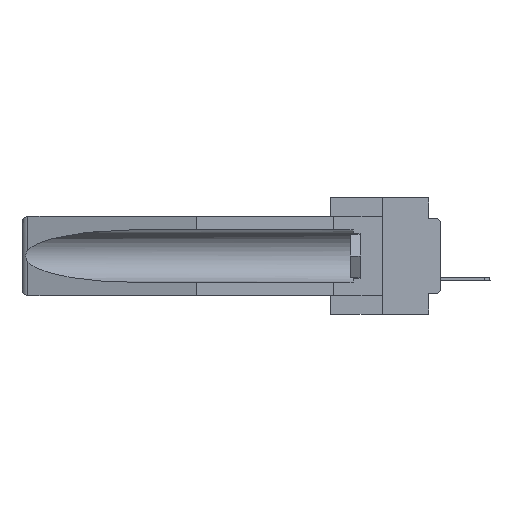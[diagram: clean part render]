
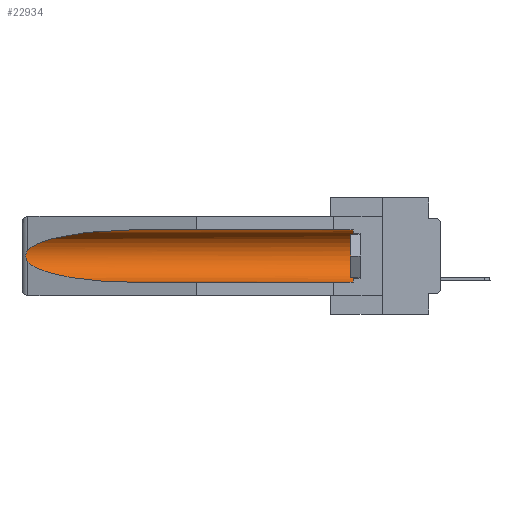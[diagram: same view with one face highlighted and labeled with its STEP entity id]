
A CAD part, left-side view. The second image highlights one B-rep face of the part: STEP entity #22934.
In plain terms, the highlighted cylindrical face has radius 2.857 mm (diameter 5.715 mm), a partial arc.
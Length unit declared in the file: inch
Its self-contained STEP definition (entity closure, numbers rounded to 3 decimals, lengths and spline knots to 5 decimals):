
#300 = CARTESIAN_POINT ( 'NONE',  ( 0.2675, 1.53308, -0.16763 ) ) ;
#750 = DIRECTION ( 'NONE',  ( 0., 0., 1. ) ) ;
#2092 = DIRECTION ( 'NONE',  ( 0., 1., 0. ) ) ;
#3161 = CARTESIAN_POINT ( 'NONE',  ( 0.2673, 1.53269, -0.17917 ) ) ;
#3666 = CARTESIAN_POINT ( 'NONE',  ( 0.26654, 1.53092, -0.15636 ) ) ;
#3973 = CARTESIAN_POINT ( 'NONE',  ( 0.21114, 1.30732, -0.284 ) ) ;
#4116 = VECTOR ( 'NONE', #8752, 39.37008 ) ;
#5172 = ORIENTED_EDGE ( 'NONE', *, *, #27428, .F. ) ;
#6545 = CARTESIAN_POINT ( 'NONE',  ( 0.26597, 1.5296, -0.19026 ) ) ;
#8145 = AXIS2_PLACEMENT_3D ( 'NONE', #26510, #17814, #750 ) ;
#8363 = ORIENTED_EDGE ( 'NONE', *, *, #35321, .T. ) ;
#8752 = DIRECTION ( 'NONE',  ( 0., 1., 0. ) ) ;
#10438 = CARTESIAN_POINT ( 'NONE',  ( 0.26537, 1.52718, -0.14972 ) ) ;
#11180 = CARTESIAN_POINT ( 'NONE',  ( 0.155, 0.126, -0.284 ) ) ;
#11376 = EDGE_CURVE ( 'NONE', #19809, #11511, #11551, .T. ) ;
#11491 = VERTEX_POINT ( 'NONE', #33739 ) ;
#11511 = VERTEX_POINT ( 'NONE', #22218 ) ;
#11551 =( BOUNDED_CURVE ( )  B_SPLINE_CURVE ( 3, ( #33262, #36137, #21859, #10438 ),
 .UNSPECIFIED., .F., .F. ) 
 B_SPLINE_CURVE_WITH_KNOTS ( ( 4, 4 ),
 ( 4.71239, 6.08839 ),
 .UNSPECIFIED. ) 
 CURVE ( )  GEOMETRIC_REPRESENTATION_ITEM ( )  RATIONAL_B_SPLINE_CURVE ( ( 1., 0.848, 0.848, 1. ) ) 
 REPRESENTATION_ITEM ( '' )  );
#12592 = CARTESIAN_POINT ( 'NONE',  ( 0.25451, 1.48313, -0.24835 ) ) ;
#12734 =( BOUNDED_CURVE ( )  B_SPLINE_CURVE ( 3, ( #32417, #12592, #3973, #29912 ),
 .UNSPECIFIED., .F., .F. ) 
 B_SPLINE_CURVE_WITH_KNOTS ( ( 4, 4 ),
 ( 0.1948, 1.5708 ),
 .UNSPECIFIED. ) 
 CURVE ( )  GEOMETRIC_REPRESENTATION_ITEM ( )  RATIONAL_B_SPLINE_CURVE ( ( 1., 0.848, 0.848, 1. ) ) 
 REPRESENTATION_ITEM ( '' )  );
#12926 = VERTEX_POINT ( 'NONE', #34328 ) ;
#13535 = CARTESIAN_POINT ( 'NONE',  ( 0.155, -0.30754, -0.059 ) ) ;
#14119 = VERTEX_POINT ( 'NONE', #20890 ) ;
#14745 = CARTESIAN_POINT ( 'NONE',  ( 0.26597, 1.52961, -0.15275 ) ) ;
#14881 = CARTESIAN_POINT ( 'NONE',  ( 0.26655, 1.53094, -0.18657 ) ) ;
#16015 = ORIENTED_EDGE ( 'NONE', *, *, #17684, .T. ) ;
#16871 = LINE ( 'NONE', #13535, #22609 ) ;
#17504 = EDGE_LOOP ( 'NONE', ( #25934, #35604, #16015, #5172, #17591, #8363 ) ) ;
#17591 = ORIENTED_EDGE ( 'NONE', *, *, #36355, .T. ) ;
#17625 = CARTESIAN_POINT ( 'NONE',  ( 0.26537, 1.52718, -0.19328 ) ) ;
#17684 = EDGE_CURVE ( 'NONE', #12926, #11491, #12734, .T. ) ;
#17814 = DIRECTION ( 'NONE',  ( 0., -1., 0. ) ) ;
#19809 = VERTEX_POINT ( 'NONE', #33232 ) ;
#20115 = LINE ( 'NONE', #27260, #4116 ) ;
#20890 = CARTESIAN_POINT ( 'NONE',  ( 0.155, 0.126, -0.059 ) ) ;
#21670 = CIRCLE ( 'NONE', #8145, 0.1125 ) ;
#21859 = CARTESIAN_POINT ( 'NONE',  ( 0.25451, 1.48313, -0.09465 ) ) ;
#22218 = CARTESIAN_POINT ( 'NONE',  ( 0.26537, 1.52718, -0.14972 ) ) ;
#22609 = VECTOR ( 'NONE', #2092, 39.37008 ) ;
#22934 = ADVANCED_FACE ( 'NONE', ( #25501 ), #28651, .F. ) ;
#23384 = DIRECTION ( 'NONE',  ( 0., 0., 1. ) ) ;
#25501 = FACE_OUTER_BOUND ( 'NONE', #17504, .T. ) ;
#25934 = ORIENTED_EDGE ( 'NONE', *, *, #11376, .T. ) ;
#26053 = CARTESIAN_POINT ( 'NONE',  ( 0.2675, 1.53308, -0.17534 ) ) ;
#26510 = CARTESIAN_POINT ( 'NONE',  ( 0.155, 0.126, -0.1715 ) ) ;
#26935 = VERTEX_POINT ( 'NONE', #11180 ) ;
#27260 = CARTESIAN_POINT ( 'NONE',  ( 0.155, -0.30754, -0.284 ) ) ;
#27428 = EDGE_CURVE ( 'NONE', #26935, #11491, #20115, .T. ) ;
#27557 = EDGE_CURVE ( 'NONE', #11511, #12926, #36956, .T. ) ;
#28651 = CYLINDRICAL_SURFACE ( 'NONE', #28770, 0.1125 ) ;
#28770 = AXIS2_PLACEMENT_3D ( 'NONE', #31783, #31915, #23384 ) ;
#29912 = CARTESIAN_POINT ( 'NONE',  ( 0.155, 1.07973, -0.284 ) ) ;
#31582 = CARTESIAN_POINT ( 'NONE',  ( 0.2673, 1.5327, -0.16383 ) ) ;
#31783 = CARTESIAN_POINT ( 'NONE',  ( 0.155, -0.30754, -0.1715 ) ) ;
#31915 = DIRECTION ( 'NONE',  ( 0., 1., 0. ) ) ;
#32417 = CARTESIAN_POINT ( 'NONE',  ( 0.26537, 1.52718, -0.19328 ) ) ;
#33232 = CARTESIAN_POINT ( 'NONE',  ( 0.155, 1.07973, -0.059 ) ) ;
#33262 = CARTESIAN_POINT ( 'NONE',  ( 0.155, 1.07973, -0.059 ) ) ;
#33739 = CARTESIAN_POINT ( 'NONE',  ( 0.155, 1.07973, -0.284 ) ) ;
#34328 = CARTESIAN_POINT ( 'NONE',  ( 0.26537, 1.52718, -0.19328 ) ) ;
#34580 = CARTESIAN_POINT ( 'NONE',  ( 0.26537, 1.52718, -0.14972 ) ) ;
#35321 = EDGE_CURVE ( 'NONE', #14119, #19809, #16871, .T. ) ;
#35604 = ORIENTED_EDGE ( 'NONE', *, *, #27557, .T. ) ;
#36137 = CARTESIAN_POINT ( 'NONE',  ( 0.21114, 1.30732, -0.059 ) ) ;
#36355 = EDGE_CURVE ( 'NONE', #26935, #14119, #21670, .T. ) ;
#36956 = B_SPLINE_CURVE_WITH_KNOTS ( 'NONE', 3,
 ( #34580, #14745, #3666, #31582, #300, #26053, #3161, #14881, #6545, #17625 ),
 .UNSPECIFIED., .F., .F.,
 ( 4, 2, 2, 2, 4 ),
 ( 0., 0.00029, 0.00058, 0.00087, 0.00117 ),
 .UNSPECIFIED. ) ;
